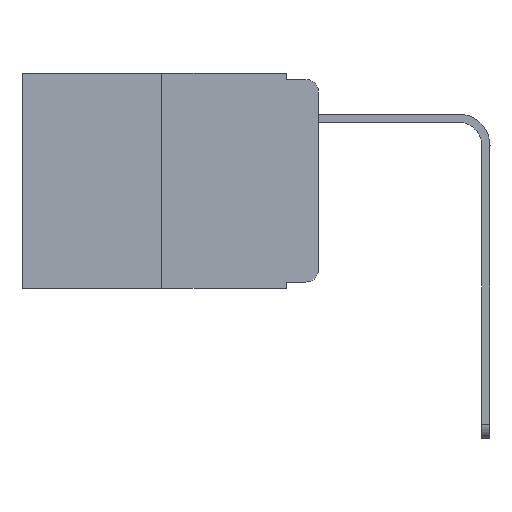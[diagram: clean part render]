
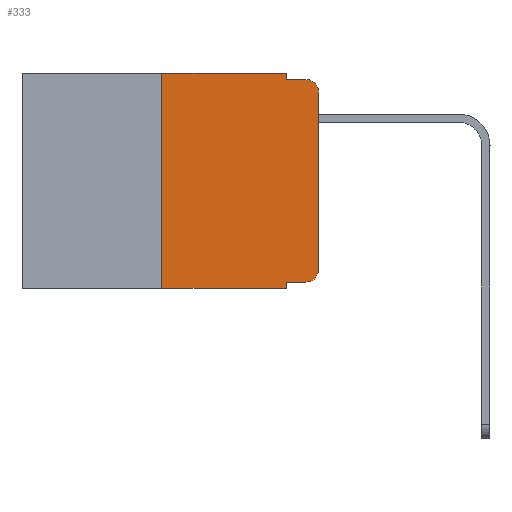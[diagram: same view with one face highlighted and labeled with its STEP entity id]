
A CAD part, left-side view. The second image highlights one B-rep face of the part: STEP entity #333.
In plain terms, the highlighted planar face has unit normal (-1, 0, 0).
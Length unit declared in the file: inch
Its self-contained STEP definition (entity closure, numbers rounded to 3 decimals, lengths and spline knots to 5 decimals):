
#333 = ADVANCED_FACE ( 'NONE', ( #5898 ), #15507, .F. ) ;
#471 = DIRECTION ( 'NONE',  ( 0., -1., 0. ) ) ;
#622 = EDGE_LOOP ( 'NONE', ( #23403, #23706, #7053, #18230, #9977, #14265, #23704, #5732, #11515, #10581 ) ) ;
#741 = EDGE_CURVE ( 'NONE', #19092, #23809, #22850, .T. ) ;
#1346 = VERTEX_POINT ( 'NONE', #5396 ) ;
#1993 = CARTESIAN_POINT ( 'NONE',  ( 0., 0.051, 0. ) ) ;
#2075 = DIRECTION ( 'NONE',  ( 0., 0., -1. ) ) ;
#2103 = VECTOR ( 'NONE', #5846, 39.37008 ) ;
#2279 = VECTOR ( 'NONE', #4124, 39.37008 ) ;
#2394 = CARTESIAN_POINT ( 'NONE',  ( 0., 0.02, -0.313 ) ) ;
#2464 = EDGE_CURVE ( 'NONE', #1346, #8705, #9147, .T. ) ;
#2679 = VECTOR ( 'NONE', #23431, 39.37008 ) ;
#3237 = AXIS2_PLACEMENT_3D ( 'NONE', #15420, #21382, #3895 ) ;
#3306 = EDGE_CURVE ( 'NONE', #16096, #15640, #24819, .T. ) ;
#3638 = EDGE_CURVE ( 'NONE', #17702, #8404, #18089, .T. ) ;
#3780 = CARTESIAN_POINT ( 'NONE',  ( 0., 0.051, -0.01 ) ) ;
#3895 = DIRECTION ( 'NONE',  ( 0., 0., -1. ) ) ;
#4124 = DIRECTION ( 'NONE',  ( 0., 0., -1. ) ) ;
#4506 = LINE ( 'NONE', #1993, #22667 ) ;
#5396 = CARTESIAN_POINT ( 'NONE',  ( 0., 0.25, 0. ) ) ;
#5482 = CARTESIAN_POINT ( 'NONE',  ( 0., 0.051, -0.343 ) ) ;
#5641 = DIRECTION ( 'NONE',  ( 0., -1., 0. ) ) ;
#5732 = ORIENTED_EDGE ( 'NONE', *, *, #17464, .F. ) ;
#5846 = DIRECTION ( 'NONE',  ( 0., -1., 0. ) ) ;
#5898 = FACE_OUTER_BOUND ( 'NONE', #622, .T. ) ;
#6496 = VECTOR ( 'NONE', #20386, 39.37008 ) ;
#6840 = EDGE_CURVE ( 'NONE', #23516, #15731, #19197, .T. ) ;
#6886 = DIRECTION ( 'NONE',  ( 0., 0., 1. ) ) ;
#7053 = ORIENTED_EDGE ( 'NONE', *, *, #741, .F. ) ;
#7549 = CARTESIAN_POINT ( 'NONE',  ( 0., 0.051, -0.333 ) ) ;
#7641 = AXIS2_PLACEMENT_3D ( 'NONE', #2394, #17917, #15873 ) ;
#7693 = CARTESIAN_POINT ( 'NONE',  ( 0., 0.051, -0.01 ) ) ;
#8281 = AXIS2_PLACEMENT_3D ( 'NONE', #16722, #18422, #24393 ) ;
#8352 = LINE ( 'NONE', #19332, #2279 ) ;
#8404 = VERTEX_POINT ( 'NONE', #15560 ) ;
#8487 = CARTESIAN_POINT ( 'NONE',  ( 0., 0.051, -0.333 ) ) ;
#8639 = CARTESIAN_POINT ( 'NONE',  ( 0., 0.02, -0.01 ) ) ;
#8705 = VERTEX_POINT ( 'NONE', #22211 ) ;
#8882 = VECTOR ( 'NONE', #6886, 39.37008 ) ;
#9147 = LINE ( 'NONE', #25023, #9755 ) ;
#9755 = VECTOR ( 'NONE', #5641, 39.37008 ) ;
#9840 = EDGE_CURVE ( 'NONE', #8404, #23809, #24817, .T. ) ;
#9977 = ORIENTED_EDGE ( 'NONE', *, *, #2464, .F. ) ;
#10390 = EDGE_CURVE ( 'NONE', #8705, #19092, #4506, .T. ) ;
#10581 = ORIENTED_EDGE ( 'NONE', *, *, #20293, .T. ) ;
#11515 = ORIENTED_EDGE ( 'NONE', *, *, #6840, .T. ) ;
#12997 = EDGE_CURVE ( 'NONE', #16096, #1346, #13645, .T. ) ;
#13408 = VECTOR ( 'NONE', #471, 39.37008 ) ;
#13645 = LINE ( 'NONE', #22540, #8882 ) ;
#14265 = ORIENTED_EDGE ( 'NONE', *, *, #12997, .F. ) ;
#15000 = CARTESIAN_POINT ( 'NONE',  ( 0., 0., 0. ) ) ;
#15420 = CARTESIAN_POINT ( 'NONE',  ( 0., 0.473, 0. ) ) ;
#15507 = PLANE ( 'NONE',  #3237 ) ;
#15560 = CARTESIAN_POINT ( 'NONE',  ( 0., 0., -0.03 ) ) ;
#15640 = VERTEX_POINT ( 'NONE', #5482 ) ;
#15731 = VERTEX_POINT ( 'NONE', #23183 ) ;
#15873 = DIRECTION ( 'NONE',  ( 0., 0., -1. ) ) ;
#16096 = VERTEX_POINT ( 'NONE', #24889 ) ;
#16422 = CARTESIAN_POINT ( 'NONE',  ( 0., 0., -0.313 ) ) ;
#16722 = CARTESIAN_POINT ( 'NONE',  ( 0., 0.02, -0.03 ) ) ;
#17464 = EDGE_CURVE ( 'NONE', #23516, #15640, #8352, .T. ) ;
#17702 = VERTEX_POINT ( 'NONE', #16422 ) ;
#17917 = DIRECTION ( 'NONE',  ( -1., 0., 0. ) ) ;
#18089 = LINE ( 'NONE', #15000, #2679 ) ;
#18230 = ORIENTED_EDGE ( 'NONE', *, *, #10390, .F. ) ;
#18422 = DIRECTION ( 'NONE',  ( -1., 0., 0. ) ) ;
#18766 = CARTESIAN_POINT ( 'NONE',  ( 0., 0.473, -0.343 ) ) ;
#19092 = VERTEX_POINT ( 'NONE', #7693 ) ;
#19197 = LINE ( 'NONE', #8487, #6496 ) ;
#19332 = CARTESIAN_POINT ( 'NONE',  ( 0., 0.051, 0. ) ) ;
#20293 = EDGE_CURVE ( 'NONE', #15731, #17702, #21292, .T. ) ;
#20386 = DIRECTION ( 'NONE',  ( 0., -1., 0. ) ) ;
#21292 = CIRCLE ( 'NONE', #7641, 0.02 ) ;
#21382 = DIRECTION ( 'NONE',  ( 1., 0., 0. ) ) ;
#22211 = CARTESIAN_POINT ( 'NONE',  ( 0., 0.051, 0. ) ) ;
#22540 = CARTESIAN_POINT ( 'NONE',  ( 0., 0.25, 0. ) ) ;
#22667 = VECTOR ( 'NONE', #2075, 39.37008 ) ;
#22850 = LINE ( 'NONE', #3780, #13408 ) ;
#23183 = CARTESIAN_POINT ( 'NONE',  ( 0., 0.02, -0.333 ) ) ;
#23403 = ORIENTED_EDGE ( 'NONE', *, *, #3638, .T. ) ;
#23431 = DIRECTION ( 'NONE',  ( 0., 0., 1. ) ) ;
#23516 = VERTEX_POINT ( 'NONE', #7549 ) ;
#23704 = ORIENTED_EDGE ( 'NONE', *, *, #3306, .T. ) ;
#23706 = ORIENTED_EDGE ( 'NONE', *, *, #9840, .T. ) ;
#23809 = VERTEX_POINT ( 'NONE', #8639 ) ;
#24393 = DIRECTION ( 'NONE',  ( 0., 0., -1. ) ) ;
#24817 = CIRCLE ( 'NONE', #8281, 0.02 ) ;
#24819 = LINE ( 'NONE', #18766, #2103 ) ;
#24889 = CARTESIAN_POINT ( 'NONE',  ( 0., 0.25, -0.343 ) ) ;
#25023 = CARTESIAN_POINT ( 'NONE',  ( 0., 0.473, 0. ) ) ;
